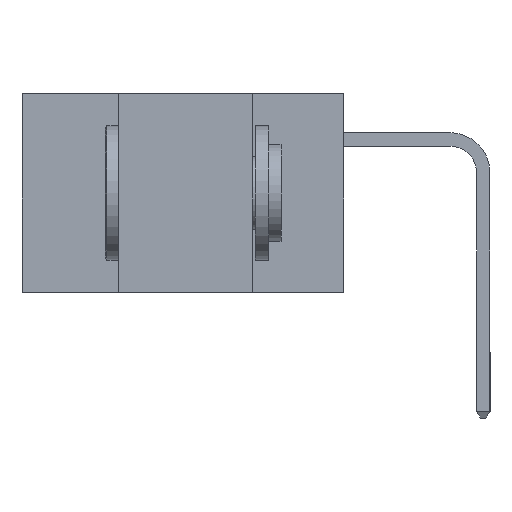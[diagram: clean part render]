
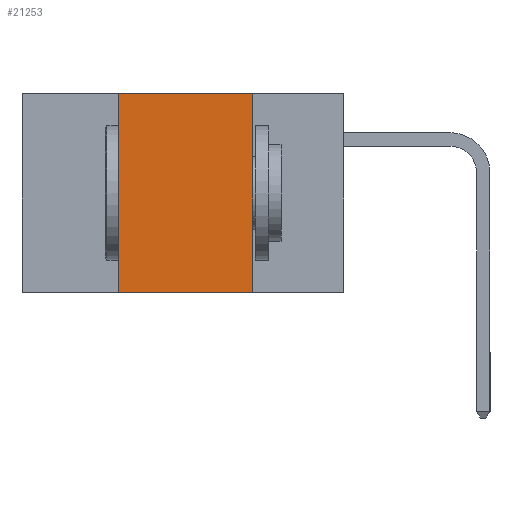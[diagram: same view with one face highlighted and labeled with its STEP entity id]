
A CAD part, left-side view. The second image highlights one B-rep face of the part: STEP entity #21253.
In plain terms, the highlighted planar face has unit normal (-1, 0, 0).
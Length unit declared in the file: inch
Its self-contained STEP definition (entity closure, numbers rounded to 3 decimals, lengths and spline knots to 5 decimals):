
#604 = DIRECTION ( 'NONE',  ( 1., 0., 0. ) ) ;
#809 = ORIENTED_EDGE ( 'NONE', *, *, #2696, .T. ) ;
#824 = EDGE_LOOP ( 'NONE', ( #1493, #15467, #30280, #809 ) ) ;
#1244 = VECTOR ( 'NONE', #26406, 39.37008 ) ;
#1493 = ORIENTED_EDGE ( 'NONE', *, *, #6972, .F. ) ;
#2696 = EDGE_CURVE ( 'NONE', #29409, #21121, #7969, .T. ) ;
#3284 = CARTESIAN_POINT ( 'NONE',  ( 0., 0.6, 0. ) ) ;
#3635 = DIRECTION ( 'NONE',  ( 0., 0., -1. ) ) ;
#5590 = DIRECTION ( 'NONE',  ( 0., 0., -1. ) ) ;
#5717 = VERTEX_POINT ( 'NONE', #26073 ) ;
#5896 = LINE ( 'NONE', #6288, #9821 ) ;
#6288 = CARTESIAN_POINT ( 'NONE',  ( 0., 0.17, 0. ) ) ;
#6972 = EDGE_CURVE ( 'NONE', #5717, #21121, #5896, .T. ) ;
#7969 = LINE ( 'NONE', #18143, #1244 ) ;
#8027 = CARTESIAN_POINT ( 'NONE',  ( 0., 0.42, 0. ) ) ;
#8153 = VECTOR ( 'NONE', #14709, 39.37008 ) ;
#8232 = CARTESIAN_POINT ( 'NONE',  ( 0., 0.6, 0. ) ) ;
#9821 = VECTOR ( 'NONE', #3635, 39.37008 ) ;
#10432 = CARTESIAN_POINT ( 'NONE',  ( 0., 0.17, -0.37 ) ) ;
#10513 = LINE ( 'NONE', #14488, #8153 ) ;
#13492 = PLANE ( 'NONE',  #21491 ) ;
#14488 = CARTESIAN_POINT ( 'NONE',  ( 0., 0.42, 0. ) ) ;
#14709 = DIRECTION ( 'NONE',  ( 0., 0., 1. ) ) ;
#15467 = ORIENTED_EDGE ( 'NONE', *, *, #26662, .F. ) ;
#16100 = LINE ( 'NONE', #3284, #22781 ) ;
#17385 = FACE_OUTER_BOUND ( 'NONE', #824, .T. ) ;
#18143 = CARTESIAN_POINT ( 'NONE',  ( 0., 0.6, -0.37 ) ) ;
#21121 = VERTEX_POINT ( 'NONE', #10432 ) ;
#21253 = ADVANCED_FACE ( 'NONE', ( #17385 ), #13492, .F. ) ;
#21491 = AXIS2_PLACEMENT_3D ( 'NONE', #8232, #604, #5590 ) ;
#22608 = CARTESIAN_POINT ( 'NONE',  ( 0., 0.42, -0.37 ) ) ;
#22781 = VECTOR ( 'NONE', #28555, 39.37008 ) ;
#26073 = CARTESIAN_POINT ( 'NONE',  ( 0., 0.17, 0. ) ) ;
#26406 = DIRECTION ( 'NONE',  ( 0., -1., 0. ) ) ;
#26662 = EDGE_CURVE ( 'NONE', #31127, #5717, #16100, .T. ) ;
#27412 = EDGE_CURVE ( 'NONE', #29409, #31127, #10513, .T. ) ;
#28555 = DIRECTION ( 'NONE',  ( 0., -1., 0. ) ) ;
#29409 = VERTEX_POINT ( 'NONE', #22608 ) ;
#30280 = ORIENTED_EDGE ( 'NONE', *, *, #27412, .F. ) ;
#31127 = VERTEX_POINT ( 'NONE', #8027 ) ;
